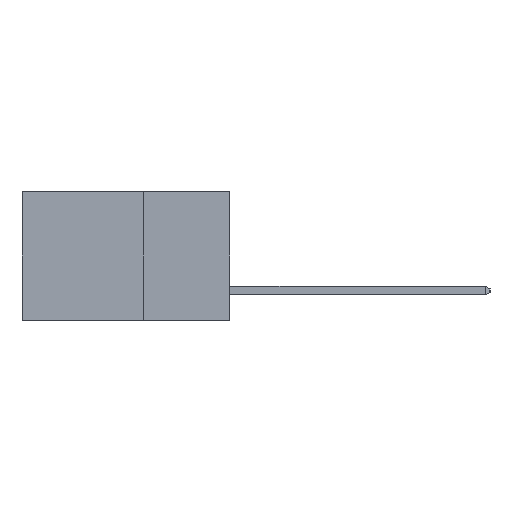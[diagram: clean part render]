
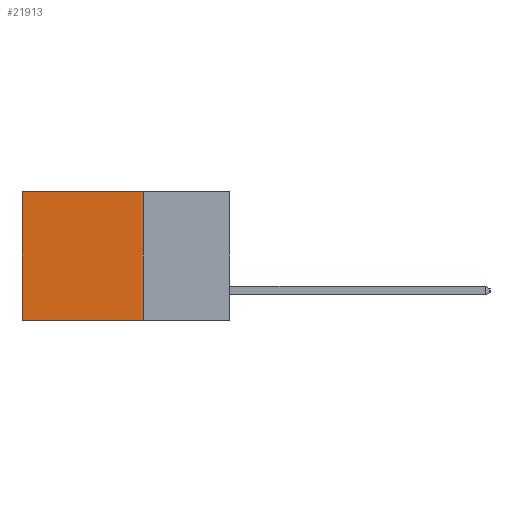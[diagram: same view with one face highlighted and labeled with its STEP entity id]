
A CAD part, left-side view. The second image highlights one B-rep face of the part: STEP entity #21913.
In plain terms, the highlighted planar face has unit normal (-1, 0, 0).
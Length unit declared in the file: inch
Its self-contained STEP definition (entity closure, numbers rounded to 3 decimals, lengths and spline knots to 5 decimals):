
#116 = AXIS2_PLACEMENT_3D ( 'NONE', #17353, #13169, #27893 ) ;
#1658 = DIRECTION ( 'NONE',  ( 0., 1., 0. ) ) ;
#3399 = CARTESIAN_POINT ( 'NONE',  ( 0.298, 0.25, 0. ) ) ;
#4095 = VECTOR ( 'NONE', #4882, 39.37008 ) ;
#4882 = DIRECTION ( 'NONE',  ( 0., 0., -1. ) ) ;
#5617 = CARTESIAN_POINT ( 'NONE',  ( 0.298, 0.6, 0. ) ) ;
#6212 = VECTOR ( 'NONE', #26009, 39.37008 ) ;
#7202 = CARTESIAN_POINT ( 'NONE',  ( 0.298, 0.6, -0.37 ) ) ;
#9013 = CARTESIAN_POINT ( 'NONE',  ( 0.298, 0.25, 0. ) ) ;
#9696 = CARTESIAN_POINT ( 'NONE',  ( 0.298, 0.25, -0.37 ) ) ;
#12914 = VERTEX_POINT ( 'NONE', #3399 ) ;
#13039 = ORIENTED_EDGE ( 'NONE', *, *, #26548, .F. ) ;
#13169 = DIRECTION ( 'NONE',  ( 1., 0., 0. ) ) ;
#13382 = EDGE_CURVE ( 'NONE', #12914, #19083, #15759, .T. ) ;
#14283 = VECTOR ( 'NONE', #1658, 39.37008 ) ;
#14904 = CARTESIAN_POINT ( 'NONE',  ( 0.298, 0.25, -0.37 ) ) ;
#15759 = LINE ( 'NONE', #22156, #4095 ) ;
#16316 = CARTESIAN_POINT ( 'NONE',  ( 0.298, 0.6, 0. ) ) ;
#16341 = VERTEX_POINT ( 'NONE', #16316 ) ;
#17235 = EDGE_CURVE ( 'NONE', #12914, #16341, #18402, .T. ) ;
#17353 = CARTESIAN_POINT ( 'NONE',  ( 0.298, 0.25, 0. ) ) ;
#17481 = EDGE_LOOP ( 'NONE', ( #23681, #13039, #24768, #19550 ) ) ;
#18402 = LINE ( 'NONE', #9013, #6212 ) ;
#18706 = DIRECTION ( 'NONE',  ( 0., 0., -1. ) ) ;
#19083 = VERTEX_POINT ( 'NONE', #9696 ) ;
#19550 = ORIENTED_EDGE ( 'NONE', *, *, #17235, .T. ) ;
#21901 = VECTOR ( 'NONE', #18706, 39.37008 ) ;
#21913 = ADVANCED_FACE ( 'NONE', ( #22496 ), #27796, .F. ) ;
#22156 = CARTESIAN_POINT ( 'NONE',  ( 0.298, 0.25, 0. ) ) ;
#22496 = FACE_OUTER_BOUND ( 'NONE', #17481, .T. ) ;
#23681 = ORIENTED_EDGE ( 'NONE', *, *, #26441, .T. ) ;
#24194 = LINE ( 'NONE', #14904, #14283 ) ;
#24768 = ORIENTED_EDGE ( 'NONE', *, *, #13382, .F. ) ;
#26009 = DIRECTION ( 'NONE',  ( 0., 1., 0. ) ) ;
#26441 = EDGE_CURVE ( 'NONE', #16341, #27319, #27448, .T. ) ;
#26548 = EDGE_CURVE ( 'NONE', #19083, #27319, #24194, .T. ) ;
#27319 = VERTEX_POINT ( 'NONE', #7202 ) ;
#27448 = LINE ( 'NONE', #5617, #21901 ) ;
#27796 = PLANE ( 'NONE',  #116 ) ;
#27893 = DIRECTION ( 'NONE',  ( 0., 0., -1. ) ) ;
